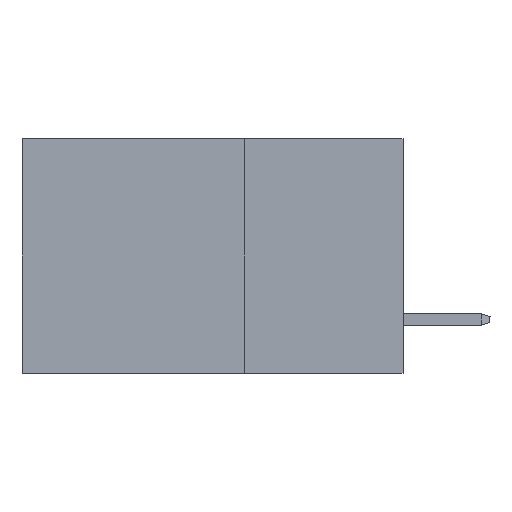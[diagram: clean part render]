
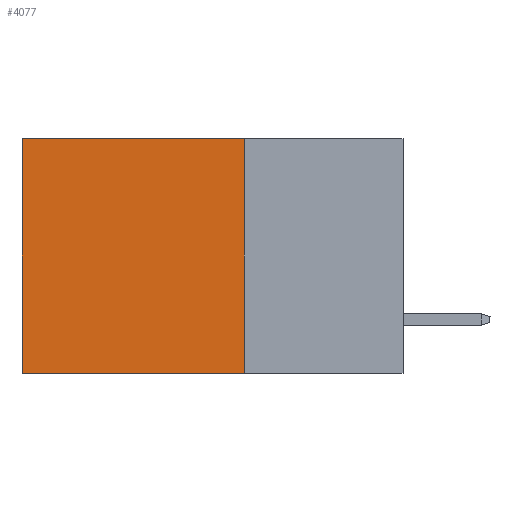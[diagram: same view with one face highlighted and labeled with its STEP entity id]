
A CAD part, left-side view. The second image highlights one B-rep face of the part: STEP entity #4077.
In plain terms, the highlighted planar face has unit normal (-1, 0, 0).
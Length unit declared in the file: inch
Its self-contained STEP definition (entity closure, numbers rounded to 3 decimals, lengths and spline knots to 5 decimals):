
#339 = DIRECTION ( 'NONE',  ( 0., 0., -1. ) ) ;
#483 = ORIENTED_EDGE ( 'NONE', *, *, #8140, .F. ) ;
#571 = DIRECTION ( 'NONE',  ( 0., 1., 0. ) ) ;
#3308 = VECTOR ( 'NONE', #10090, 39.37008 ) ;
#3373 = DIRECTION ( 'NONE',  ( 1., 0., 0. ) ) ;
#4077 = ADVANCED_FACE ( 'NONE', ( #25622 ), #20557, .F. ) ;
#4960 = CARTESIAN_POINT ( 'NONE',  ( 0.2875, 0.25, 0. ) ) ;
#6359 = LINE ( 'NONE', #16494, #3308 ) ;
#6555 = EDGE_CURVE ( 'NONE', #20446, #23400, #18001, .T. ) ;
#7074 = VECTOR ( 'NONE', #571, 39.37008 ) ;
#7204 = CARTESIAN_POINT ( 'NONE',  ( 0.2875, 0.25, 0. ) ) ;
#8140 = EDGE_CURVE ( 'NONE', #19459, #23484, #24389, .T. ) ;
#10090 = DIRECTION ( 'NONE',  ( 0., 1., 0. ) ) ;
#11305 = ORIENTED_EDGE ( 'NONE', *, *, #30351, .F. ) ;
#12980 = CARTESIAN_POINT ( 'NONE',  ( 0.2875, 0.25, -0.37 ) ) ;
#15317 = DIRECTION ( 'NONE',  ( 0., 0., -1. ) ) ;
#15446 = LINE ( 'NONE', #12980, #7074 ) ;
#15791 = CARTESIAN_POINT ( 'NONE',  ( 0.2875, 0.25, 0. ) ) ;
#16494 = CARTESIAN_POINT ( 'NONE',  ( 0.2875, 0.25, 0. ) ) ;
#18001 = LINE ( 'NONE', #18315, #21157 ) ;
#18315 = CARTESIAN_POINT ( 'NONE',  ( 0.2875, 0.6, 0. ) ) ;
#19459 = VERTEX_POINT ( 'NONE', #4960 ) ;
#20446 = VERTEX_POINT ( 'NONE', #31324 ) ;
#20557 = PLANE ( 'NONE',  #27829 ) ;
#21157 = VECTOR ( 'NONE', #339, 39.37008 ) ;
#21471 = EDGE_LOOP ( 'NONE', ( #25421, #11305, #483, #31604 ) ) ;
#22230 = DIRECTION ( 'NONE',  ( 0., 0., -1. ) ) ;
#22961 = CARTESIAN_POINT ( 'NONE',  ( 0.2875, 0.6, -0.37 ) ) ;
#23400 = VERTEX_POINT ( 'NONE', #22961 ) ;
#23484 = VERTEX_POINT ( 'NONE', #29453 ) ;
#24389 = LINE ( 'NONE', #7204, #25133 ) ;
#25133 = VECTOR ( 'NONE', #22230, 39.37008 ) ;
#25421 = ORIENTED_EDGE ( 'NONE', *, *, #6555, .T. ) ;
#25622 = FACE_OUTER_BOUND ( 'NONE', #21471, .T. ) ;
#27829 = AXIS2_PLACEMENT_3D ( 'NONE', #15791, #3373, #15317 ) ;
#28429 = EDGE_CURVE ( 'NONE', #19459, #20446, #6359, .T. ) ;
#29453 = CARTESIAN_POINT ( 'NONE',  ( 0.2875, 0.25, -0.37 ) ) ;
#30351 = EDGE_CURVE ( 'NONE', #23484, #23400, #15446, .T. ) ;
#31324 = CARTESIAN_POINT ( 'NONE',  ( 0.2875, 0.6, 0. ) ) ;
#31604 = ORIENTED_EDGE ( 'NONE', *, *, #28429, .T. ) ;
